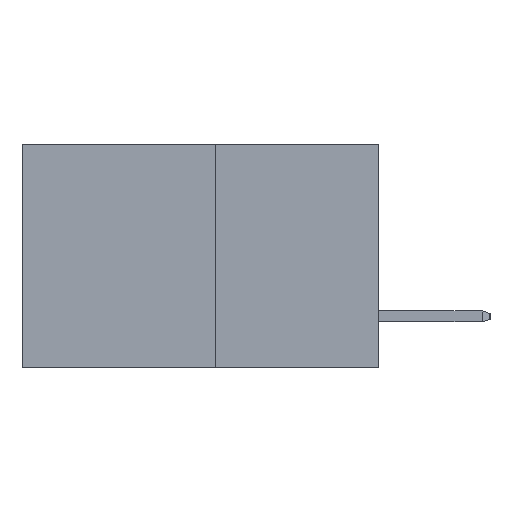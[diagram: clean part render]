
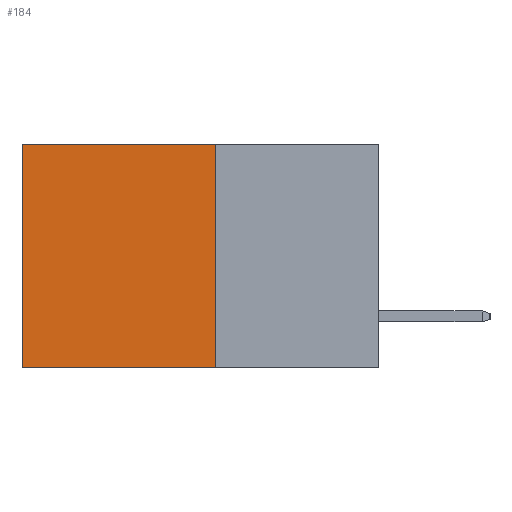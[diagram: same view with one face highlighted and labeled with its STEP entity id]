
A CAD part, left-side view. The second image highlights one B-rep face of the part: STEP entity #184.
In plain terms, the highlighted planar face has unit normal (-1, 0, 0).
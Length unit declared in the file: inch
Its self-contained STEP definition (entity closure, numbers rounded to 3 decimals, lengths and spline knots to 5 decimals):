
#184 = ADVANCED_FACE ( 'NONE', ( #12591 ), #17853, .F. ) ;
#264 = CARTESIAN_POINT ( 'NONE',  ( 0.277, 0.27, -0.37 ) ) ;
#1963 = EDGE_LOOP ( 'NONE', ( #15451, #14013, #17019, #18070 ) ) ;
#2377 = VERTEX_POINT ( 'NONE', #4583 ) ;
#3069 = CARTESIAN_POINT ( 'NONE',  ( 0.277, 0.59, 0. ) ) ;
#3622 = VECTOR ( 'NONE', #7365, 39.37008 ) ;
#4208 = VERTEX_POINT ( 'NONE', #13359 ) ;
#4583 = CARTESIAN_POINT ( 'NONE',  ( 0.277, 0.27, 0. ) ) ;
#5286 = LINE ( 'NONE', #264, #12780 ) ;
#5754 = CARTESIAN_POINT ( 'NONE',  ( 0.277, 0.27, 0. ) ) ;
#6207 = DIRECTION ( 'NONE',  ( 0., 0., -1. ) ) ;
#7105 = VERTEX_POINT ( 'NONE', #10733 ) ;
#7365 = DIRECTION ( 'NONE',  ( 0., 1., 0. ) ) ;
#8873 = EDGE_CURVE ( 'NONE', #2377, #11688, #17682, .T. ) ;
#9042 = DIRECTION ( 'NONE',  ( 0., 1., 0. ) ) ;
#9065 = EDGE_CURVE ( 'NONE', #2377, #4208, #10632, .T. ) ;
#9213 = CARTESIAN_POINT ( 'NONE',  ( 0.277, 0.27, -0.37 ) ) ;
#10470 = EDGE_CURVE ( 'NONE', #11688, #7105, #11389, .T. ) ;
#10632 = LINE ( 'NONE', #9213, #17469 ) ;
#10733 = CARTESIAN_POINT ( 'NONE',  ( 0.277, 0.59, -0.37 ) ) ;
#10984 = VECTOR ( 'NONE', #13145, 39.37008 ) ;
#11389 = LINE ( 'NONE', #11766, #10984 ) ;
#11688 = VERTEX_POINT ( 'NONE', #3069 ) ;
#11766 = CARTESIAN_POINT ( 'NONE',  ( 0.277, 0.59, -0.37 ) ) ;
#12591 = FACE_OUTER_BOUND ( 'NONE', #1963, .T. ) ;
#12780 = VECTOR ( 'NONE', #9042, 39.37008 ) ;
#13145 = DIRECTION ( 'NONE',  ( 0., 0., -1. ) ) ;
#13359 = CARTESIAN_POINT ( 'NONE',  ( 0.277, 0.27, -0.37 ) ) ;
#13940 = DIRECTION ( 'NONE',  ( 1., 0., 0. ) ) ;
#14013 = ORIENTED_EDGE ( 'NONE', *, *, #16076, .F. ) ;
#15451 = ORIENTED_EDGE ( 'NONE', *, *, #10470, .T. ) ;
#16076 = EDGE_CURVE ( 'NONE', #4208, #7105, #5286, .T. ) ;
#16582 = DIRECTION ( 'NONE',  ( 0., 0., -1. ) ) ;
#16946 = AXIS2_PLACEMENT_3D ( 'NONE', #17724, #13940, #16582 ) ;
#17019 = ORIENTED_EDGE ( 'NONE', *, *, #9065, .F. ) ;
#17469 = VECTOR ( 'NONE', #6207, 39.37008 ) ;
#17682 = LINE ( 'NONE', #5754, #3622 ) ;
#17724 = CARTESIAN_POINT ( 'NONE',  ( 0.277, 0.27, -0.37 ) ) ;
#17853 = PLANE ( 'NONE',  #16946 ) ;
#18070 = ORIENTED_EDGE ( 'NONE', *, *, #8873, .T. ) ;
